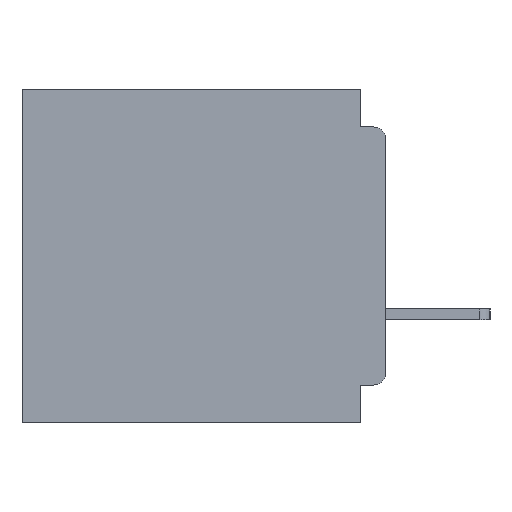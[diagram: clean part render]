
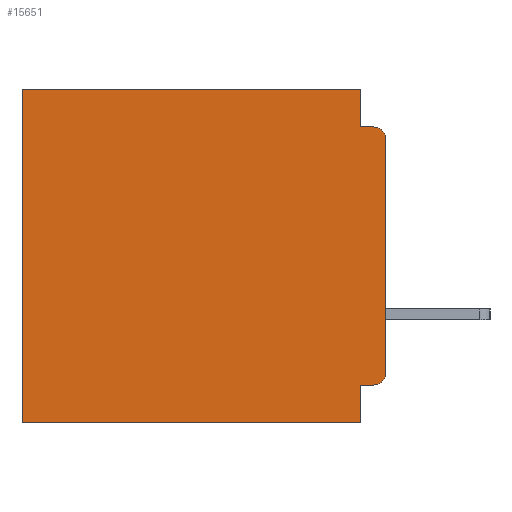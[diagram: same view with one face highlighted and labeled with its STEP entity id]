
A CAD part, left-side view. The second image highlights one B-rep face of the part: STEP entity #15651.
In plain terms, the highlighted planar face has unit normal (-1, 0, 0).
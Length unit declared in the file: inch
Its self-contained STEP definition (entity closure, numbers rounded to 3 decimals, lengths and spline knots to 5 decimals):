
#135 = ORIENTED_EDGE ( 'NONE', *, *, #8851, .T. ) ;
#361 = AXIS2_PLACEMENT_3D ( 'NONE', #54297, #1023, #46353 ) ;
#1023 = DIRECTION ( 'NONE',  ( -1., 0., 0. ) ) ;
#1758 = CARTESIAN_POINT ( 'NONE',  ( 0.3, 0., 0. ) ) ;
#2347 = EDGE_CURVE ( 'NONE', #13486, #46633, #45728, .T. ) ;
#3466 = VECTOR ( 'NONE', #49093, 39.37008 ) ;
#3917 = EDGE_CURVE ( 'NONE', #28520, #33028, #18138, .T. ) ;
#5062 = ORIENTED_EDGE ( 'NONE', *, *, #7152, .F. ) ;
#6203 = ORIENTED_EDGE ( 'NONE', *, *, #3917, .F. ) ;
#6315 = VERTEX_POINT ( 'NONE', #30369 ) ;
#6337 = CARTESIAN_POINT ( 'NONE',  ( 0.3, 0., -0.4 ) ) ;
#6641 = AXIS2_PLACEMENT_3D ( 'NONE', #6337, #36482, #10681 ) ;
#7059 = LINE ( 'NONE', #1758, #28713 ) ;
#7152 = EDGE_CURVE ( 'NONE', #23679, #46633, #39274, .T. ) ;
#7264 = VERTEX_POINT ( 'NONE', #51278 ) ;
#7384 = CARTESIAN_POINT ( 'NONE',  ( 0.3, 0.437, -0.4 ) ) ;
#8279 = ORIENTED_EDGE ( 'NONE', *, *, #2347, .T. ) ;
#8851 = EDGE_CURVE ( 'NONE', #25220, #33028, #25114, .T. ) ;
#8933 = EDGE_CURVE ( 'NONE', #13486, #50140, #52370, .T. ) ;
#10002 = EDGE_CURVE ( 'NONE', #7264, #50140, #43282, .T. ) ;
#10236 = DIRECTION ( 'NONE',  ( 0., 1., 0. ) ) ;
#10302 = CARTESIAN_POINT ( 'NONE',  ( 0.3, 0., -0.06 ) ) ;
#10681 = DIRECTION ( 'NONE',  ( 0., 0., -1. ) ) ;
#11182 = CARTESIAN_POINT ( 'NONE',  ( 0.3, 0.031, -0.045 ) ) ;
#12091 = DIRECTION ( 'NONE',  ( 0., 0., -1. ) ) ;
#13486 = VERTEX_POINT ( 'NONE', #10302 ) ;
#13835 = VECTOR ( 'NONE', #12091, 39.37008 ) ;
#15651 = ADVANCED_FACE ( 'NONE', ( #36069 ), #23352, .F. ) ;
#16483 = CARTESIAN_POINT ( 'NONE',  ( 0.3, 0.031, -0.4 ) ) ;
#16523 = EDGE_CURVE ( 'NONE', #47803, #28520, #28064, .T. ) ;
#18138 = LINE ( 'NONE', #21864, #50820 ) ;
#18765 = AXIS2_PLACEMENT_3D ( 'NONE', #23426, #53164, #27807 ) ;
#18912 = EDGE_LOOP ( 'NONE', ( #41537, #8279, #5062, #35629, #29608, #135, #6203, #34773, #32271, #38028 ) ) ;
#19061 = CARTESIAN_POINT ( 'NONE',  ( 0.3, 0., -0.355 ) ) ;
#21864 = CARTESIAN_POINT ( 'NONE',  ( 0.3, 0., -0.4 ) ) ;
#23352 = PLANE ( 'NONE',  #6641 ) ;
#23426 = CARTESIAN_POINT ( 'NONE',  ( 0.3, 0.015, -0.34 ) ) ;
#23679 = VERTEX_POINT ( 'NONE', #11182 ) ;
#24210 = EDGE_CURVE ( 'NONE', #6315, #25220, #7059, .T. ) ;
#24564 = LINE ( 'NONE', #19061, #34632 ) ;
#25052 = CARTESIAN_POINT ( 'NONE',  ( 0.3, 0., -0.045 ) ) ;
#25114 = LINE ( 'NONE', #32219, #3466 ) ;
#25220 = VERTEX_POINT ( 'NONE', #38739 ) ;
#26465 = DIRECTION ( 'NONE',  ( 0., 0., -1. ) ) ;
#27185 = CARTESIAN_POINT ( 'NONE',  ( 0.3, 0., -0.34 ) ) ;
#27807 = DIRECTION ( 'NONE',  ( 0., 0., -1. ) ) ;
#27953 = VECTOR ( 'NONE', #50552, 39.37008 ) ;
#28064 = LINE ( 'NONE', #16483, #13835 ) ;
#28520 = VERTEX_POINT ( 'NONE', #52495 ) ;
#28713 = VECTOR ( 'NONE', #10236, 39.37008 ) ;
#29608 = ORIENTED_EDGE ( 'NONE', *, *, #24210, .T. ) ;
#30369 = CARTESIAN_POINT ( 'NONE',  ( 0.3, 0.031, 0. ) ) ;
#32219 = CARTESIAN_POINT ( 'NONE',  ( 0.3, 0.437, -0.4 ) ) ;
#32271 = ORIENTED_EDGE ( 'NONE', *, *, #50234, .F. ) ;
#33028 = VERTEX_POINT ( 'NONE', #7384 ) ;
#33330 = EDGE_CURVE ( 'NONE', #6315, #23679, #43926, .T. ) ;
#34632 = VECTOR ( 'NONE', #44667, 39.37008 ) ;
#34773 = ORIENTED_EDGE ( 'NONE', *, *, #16523, .F. ) ;
#35629 = ORIENTED_EDGE ( 'NONE', *, *, #33330, .F. ) ;
#35726 = DIRECTION ( 'NONE',  ( 0., 1., 0. ) ) ;
#35836 = CARTESIAN_POINT ( 'NONE',  ( 0.3, 0.015, -0.045 ) ) ;
#36069 = FACE_OUTER_BOUND ( 'NONE', #18912, .T. ) ;
#36482 = DIRECTION ( 'NONE',  ( 1., 0., 0. ) ) ;
#37045 = DIRECTION ( 'NONE',  ( 0., 0., -1. ) ) ;
#38028 = ORIENTED_EDGE ( 'NONE', *, *, #10002, .T. ) ;
#38739 = CARTESIAN_POINT ( 'NONE',  ( 0.3, 0.437, 0. ) ) ;
#38888 = CARTESIAN_POINT ( 'NONE',  ( 0.3, 0.031, -0.355 ) ) ;
#39274 = LINE ( 'NONE', #25052, #27953 ) ;
#41149 = VECTOR ( 'NONE', #37045, 39.37008 ) ;
#41537 = ORIENTED_EDGE ( 'NONE', *, *, #8933, .F. ) ;
#42586 = VECTOR ( 'NONE', #26465, 39.37008 ) ;
#43282 = CIRCLE ( 'NONE', #18765, 0.015 ) ;
#43926 = LINE ( 'NONE', #52093, #42586 ) ;
#44667 = DIRECTION ( 'NONE',  ( 0., 1., 0. ) ) ;
#45383 = CARTESIAN_POINT ( 'NONE',  ( 0.3, 0., -0.4 ) ) ;
#45728 = CIRCLE ( 'NONE', #361, 0.015 ) ;
#46353 = DIRECTION ( 'NONE',  ( 0., 0., -1. ) ) ;
#46633 = VERTEX_POINT ( 'NONE', #35836 ) ;
#47803 = VERTEX_POINT ( 'NONE', #38888 ) ;
#49093 = DIRECTION ( 'NONE',  ( 0., 0., -1. ) ) ;
#50140 = VERTEX_POINT ( 'NONE', #27185 ) ;
#50234 = EDGE_CURVE ( 'NONE', #7264, #47803, #24564, .T. ) ;
#50552 = DIRECTION ( 'NONE',  ( 0., -1., 0. ) ) ;
#50820 = VECTOR ( 'NONE', #35726, 39.37008 ) ;
#51278 = CARTESIAN_POINT ( 'NONE',  ( 0.3, 0.015, -0.355 ) ) ;
#52093 = CARTESIAN_POINT ( 'NONE',  ( 0.3, 0.031, 0. ) ) ;
#52370 = LINE ( 'NONE', #45383, #41149 ) ;
#52495 = CARTESIAN_POINT ( 'NONE',  ( 0.3, 0.031, -0.4 ) ) ;
#53164 = DIRECTION ( 'NONE',  ( -1., 0., 0. ) ) ;
#54297 = CARTESIAN_POINT ( 'NONE',  ( 0.3, 0.015, -0.06 ) ) ;
